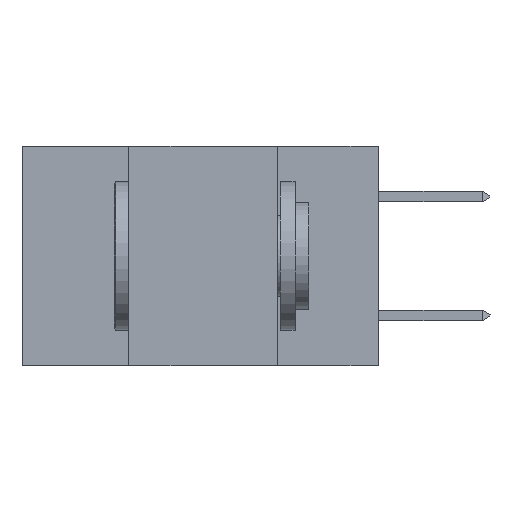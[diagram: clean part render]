
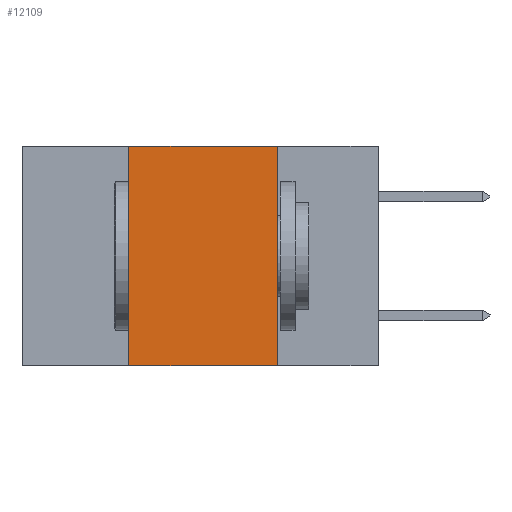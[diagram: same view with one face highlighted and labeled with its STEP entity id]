
A CAD part, left-side view. The second image highlights one B-rep face of the part: STEP entity #12109.
In plain terms, the highlighted planar face has unit normal (-1, 0, 0).
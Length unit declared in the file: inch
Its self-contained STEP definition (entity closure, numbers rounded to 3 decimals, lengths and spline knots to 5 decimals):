
#943 = LINE ( 'NONE', #29720, #14530 ) ;
#3035 = EDGE_CURVE ( 'NONE', #3088, #4803, #23296, .T. ) ;
#3088 = VERTEX_POINT ( 'NONE', #16713 ) ;
#3805 = VECTOR ( 'NONE', #19242, 39.37008 ) ;
#4803 = VERTEX_POINT ( 'NONE', #14539 ) ;
#6493 = ORIENTED_EDGE ( 'NONE', *, *, #3035, .F. ) ;
#7777 = VECTOR ( 'NONE', #23126, 39.37008 ) ;
#7923 = CARTESIAN_POINT ( 'NONE',  ( 0., 0.17, 0. ) ) ;
#10160 = CARTESIAN_POINT ( 'NONE',  ( 0., 0.6, 0. ) ) ;
#12109 = ADVANCED_FACE ( 'NONE', ( #12867 ), #20220, .F. ) ;
#12601 = VERTEX_POINT ( 'NONE', #15231 ) ;
#12736 = DIRECTION ( 'NONE',  ( 0., 0., -1. ) ) ;
#12867 = FACE_OUTER_BOUND ( 'NONE', #28397, .T. ) ;
#13905 = VERTEX_POINT ( 'NONE', #20548 ) ;
#14530 = VECTOR ( 'NONE', #14607, 39.37008 ) ;
#14539 = CARTESIAN_POINT ( 'NONE',  ( 0., 0.17, 0. ) ) ;
#14591 = LINE ( 'NONE', #7923, #7777 ) ;
#14607 = DIRECTION ( 'NONE',  ( 0., 0., 1. ) ) ;
#14934 = ORIENTED_EDGE ( 'NONE', *, *, #30053, .T. ) ;
#15231 = CARTESIAN_POINT ( 'NONE',  ( 0., 0.17, -0.37 ) ) ;
#15275 = EDGE_CURVE ( 'NONE', #4803, #12601, #14591, .T. ) ;
#16713 = CARTESIAN_POINT ( 'NONE',  ( 0., 0.42, 0. ) ) ;
#16880 = ORIENTED_EDGE ( 'NONE', *, *, #15275, .F. ) ;
#18788 = CARTESIAN_POINT ( 'NONE',  ( 0., 0.6, 0. ) ) ;
#19242 = DIRECTION ( 'NONE',  ( 0., -1., 0. ) ) ;
#19970 = DIRECTION ( 'NONE',  ( 0., -1., 0. ) ) ;
#20043 = ORIENTED_EDGE ( 'NONE', *, *, #24022, .F. ) ;
#20220 = PLANE ( 'NONE',  #32229 ) ;
#20548 = CARTESIAN_POINT ( 'NONE',  ( 0., 0.42, -0.37 ) ) ;
#23126 = DIRECTION ( 'NONE',  ( 0., 0., -1. ) ) ;
#23296 = LINE ( 'NONE', #18788, #3805 ) ;
#24022 = EDGE_CURVE ( 'NONE', #13905, #3088, #943, .T. ) ;
#27355 = LINE ( 'NONE', #27439, #32521 ) ;
#27439 = CARTESIAN_POINT ( 'NONE',  ( 0., 0.6, -0.37 ) ) ;
#27821 = DIRECTION ( 'NONE',  ( 1., 0., 0. ) ) ;
#28397 = EDGE_LOOP ( 'NONE', ( #16880, #6493, #20043, #14934 ) ) ;
#29720 = CARTESIAN_POINT ( 'NONE',  ( 0., 0.42, 0. ) ) ;
#30053 = EDGE_CURVE ( 'NONE', #13905, #12601, #27355, .T. ) ;
#32229 = AXIS2_PLACEMENT_3D ( 'NONE', #10160, #27821, #12736 ) ;
#32521 = VECTOR ( 'NONE', #19970, 39.37008 ) ;
